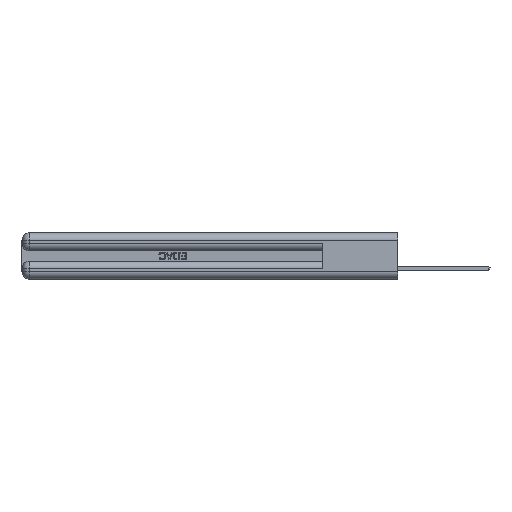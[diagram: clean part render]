
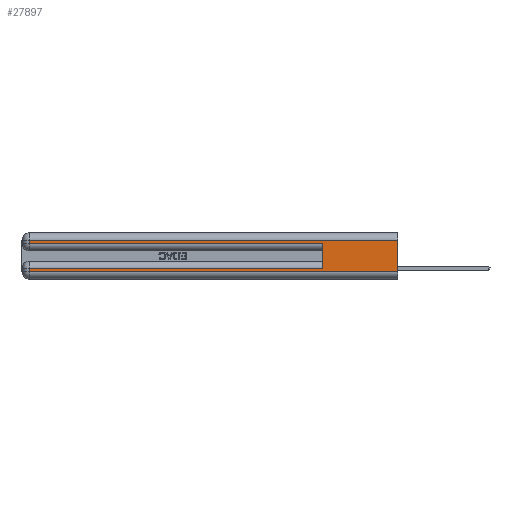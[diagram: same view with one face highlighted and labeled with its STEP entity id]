
A CAD part, left-side view. The second image highlights one B-rep face of the part: STEP entity #27897.
In plain terms, the highlighted planar face has unit normal (-1, 0, 0).
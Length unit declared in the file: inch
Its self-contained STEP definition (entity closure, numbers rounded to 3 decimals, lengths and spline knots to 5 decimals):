
#31 = ORIENTED_EDGE ( 'NONE', *, *, #1553, .T. ) ;
#887 = EDGE_CURVE ( 'NONE', #11383, #14684, #35290, .T. ) ;
#937 = DIRECTION ( 'NONE',  ( 0., 0., -1. ) ) ;
#1553 = EDGE_CURVE ( 'NONE', #26219, #14684, #14830, .T. ) ;
#1623 = CARTESIAN_POINT ( 'NONE',  ( 0., 0.6, 0.145 ) ) ;
#2321 = VECTOR ( 'NONE', #13165, 39.37008 ) ;
#2427 = EDGE_CURVE ( 'NONE', #5786, #48398, #52358, .T. ) ;
#4276 = DIRECTION ( 'NONE',  ( 0., -1., 0. ) ) ;
#4865 = DIRECTION ( 'NONE',  ( 1., 0., 0. ) ) ;
#5039 = VECTOR ( 'NONE', #51333, 39.37008 ) ;
#5753 = VECTOR ( 'NONE', #37106, 39.37008 ) ;
#5786 = VERTEX_POINT ( 'NONE', #54210 ) ;
#6548 = CARTESIAN_POINT ( 'NONE',  ( 0., 0., 0.31 ) ) ;
#7431 = CARTESIAN_POINT ( 'NONE',  ( 0., 0., 0.085 ) ) ;
#7470 = ORIENTED_EDGE ( 'NONE', *, *, #22525, .F. ) ;
#8053 = EDGE_CURVE ( 'NONE', #50619, #5786, #37277, .T. ) ;
#9206 = VECTOR ( 'NONE', #20093, 39.37008 ) ;
#9849 = VERTEX_POINT ( 'NONE', #33970 ) ;
#10436 = LINE ( 'NONE', #36683, #53288 ) ;
#10797 = EDGE_LOOP ( 'NONE', ( #7470, #41771, #41076, #31, #40995, #43527, #14872, #26243 ) ) ;
#11383 = VERTEX_POINT ( 'NONE', #18917 ) ;
#11453 = DIRECTION ( 'NONE',  ( 0., 1., 0. ) ) ;
#12469 = PLANE ( 'NONE',  #28807 ) ;
#12793 = DIRECTION ( 'NONE',  ( 0., -1., 0. ) ) ;
#13165 = DIRECTION ( 'NONE',  ( 0., 0., -1. ) ) ;
#13515 = CARTESIAN_POINT ( 'NONE',  ( 0., 2.94, 0.37 ) ) ;
#14684 = VERTEX_POINT ( 'NONE', #25246 ) ;
#14830 = LINE ( 'NONE', #33792, #41250 ) ;
#14872 = ORIENTED_EDGE ( 'NONE', *, *, #8053, .T. ) ;
#15625 = CARTESIAN_POINT ( 'NONE',  ( 0., 2.94, 0.085 ) ) ;
#16267 = DIRECTION ( 'NONE',  ( 0., 0., -1. ) ) ;
#18917 = CARTESIAN_POINT ( 'NONE',  ( 0., 0.6, 0.085 ) ) ;
#20093 = DIRECTION ( 'NONE',  ( 0., 1., 0. ) ) ;
#21123 = LINE ( 'NONE', #33002, #53421 ) ;
#22525 = EDGE_CURVE ( 'NONE', #52812, #48398, #28149, .T. ) ;
#25246 = CARTESIAN_POINT ( 'NONE',  ( 0., 0.6, 0.285 ) ) ;
#25508 = CARTESIAN_POINT ( 'NONE',  ( 0., 0., 0.06 ) ) ;
#26219 = VERTEX_POINT ( 'NONE', #30897 ) ;
#26243 = ORIENTED_EDGE ( 'NONE', *, *, #2427, .T. ) ;
#27897 = ADVANCED_FACE ( 'NONE', ( #32957 ), #12469, .F. ) ;
#28149 = LINE ( 'NONE', #32480, #5753 ) ;
#28807 = AXIS2_PLACEMENT_3D ( 'NONE', #33464, #4865, #937 ) ;
#30897 = CARTESIAN_POINT ( 'NONE',  ( 0., 2.94, 0.285 ) ) ;
#32480 = CARTESIAN_POINT ( 'NONE',  ( 0., 0., 0.37 ) ) ;
#32957 = FACE_OUTER_BOUND ( 'NONE', #10797, .T. ) ;
#33002 = CARTESIAN_POINT ( 'NONE',  ( 0., 0., 0.31 ) ) ;
#33464 = CARTESIAN_POINT ( 'NONE',  ( 0., 0., 0.37 ) ) ;
#33792 = CARTESIAN_POINT ( 'NONE',  ( 0., 0., 0.285 ) ) ;
#33970 = CARTESIAN_POINT ( 'NONE',  ( 0., 2.94, 0.31 ) ) ;
#33986 = CARTESIAN_POINT ( 'NONE',  ( 0., 0., 0.06 ) ) ;
#35290 = LINE ( 'NONE', #1623, #5039 ) ;
#36683 = CARTESIAN_POINT ( 'NONE',  ( 0., 2.94, 0.37 ) ) ;
#37106 = DIRECTION ( 'NONE',  ( 0., 0., -1. ) ) ;
#37277 = LINE ( 'NONE', #13515, #2321 ) ;
#40995 = ORIENTED_EDGE ( 'NONE', *, *, #887, .F. ) ;
#41076 = ORIENTED_EDGE ( 'NONE', *, *, #51774, .T. ) ;
#41250 = VECTOR ( 'NONE', #12793, 39.37008 ) ;
#41264 = VECTOR ( 'NONE', #4276, 39.37008 ) ;
#41771 = ORIENTED_EDGE ( 'NONE', *, *, #43626, .T. ) ;
#42768 = LINE ( 'NONE', #7431, #9206 ) ;
#43527 = ORIENTED_EDGE ( 'NONE', *, *, #43577, .T. ) ;
#43577 = EDGE_CURVE ( 'NONE', #11383, #50619, #42768, .T. ) ;
#43626 = EDGE_CURVE ( 'NONE', #52812, #9849, #21123, .T. ) ;
#48398 = VERTEX_POINT ( 'NONE', #25508 ) ;
#50619 = VERTEX_POINT ( 'NONE', #15625 ) ;
#51333 = DIRECTION ( 'NONE',  ( 0., 0., 1. ) ) ;
#51774 = EDGE_CURVE ( 'NONE', #9849, #26219, #10436, .T. ) ;
#52358 = LINE ( 'NONE', #33986, #41264 ) ;
#52812 = VERTEX_POINT ( 'NONE', #6548 ) ;
#53288 = VECTOR ( 'NONE', #16267, 39.37008 ) ;
#53421 = VECTOR ( 'NONE', #11453, 39.37008 ) ;
#54210 = CARTESIAN_POINT ( 'NONE',  ( 0., 2.94, 0.06 ) ) ;
